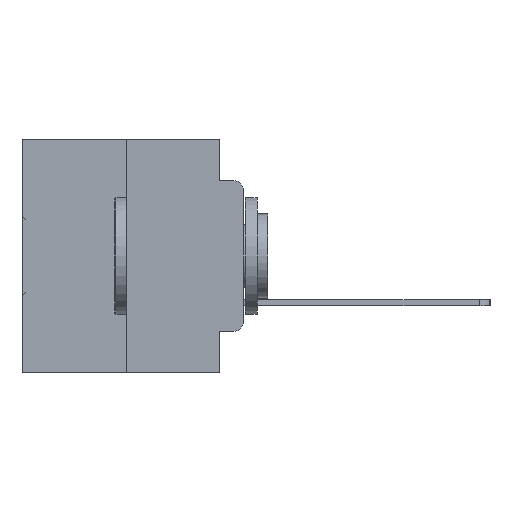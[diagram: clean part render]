
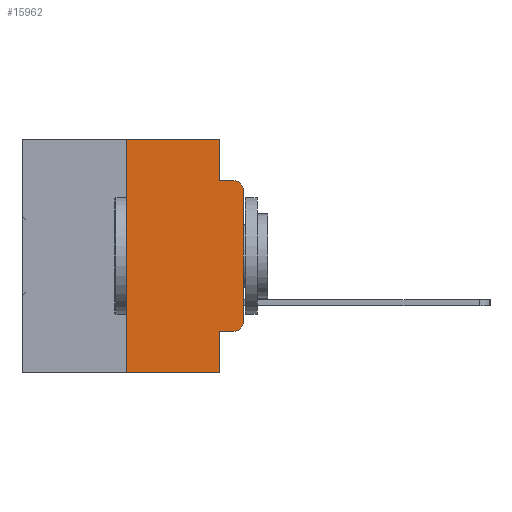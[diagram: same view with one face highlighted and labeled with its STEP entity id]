
A CAD part, left-side view. The second image highlights one B-rep face of the part: STEP entity #15962.
In plain terms, the highlighted planar face has unit normal (-1, 0, 0).
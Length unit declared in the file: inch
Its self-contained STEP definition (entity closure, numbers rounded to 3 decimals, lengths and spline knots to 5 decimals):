
#16 = CARTESIAN_POINT ( 'NONE',  ( 0., 0., 0. ) ) ;
#320 = DIRECTION ( 'NONE',  ( 0., 0., -1. ) ) ;
#1025 = PLANE ( 'NONE',  #18663 ) ;
#1897 = DIRECTION ( 'NONE',  ( 0., -1., 0. ) ) ;
#2776 = AXIS2_PLACEMENT_3D ( 'NONE', #21929, #6407, #24409 ) ;
#3374 = CIRCLE ( 'NONE', #24755, 0.02 ) ;
#3681 = CARTESIAN_POINT ( 'NONE',  ( 0., 0.473, 0. ) ) ;
#3809 = ORIENTED_EDGE ( 'NONE', *, *, #6567, .T. ) ;
#4176 = EDGE_CURVE ( 'NONE', #5156, #12579, #27733, .T. ) ;
#4270 = CARTESIAN_POINT ( 'NONE',  ( 0., 0.02, -0.0885 ) ) ;
#4366 = VECTOR ( 'NONE', #25576, 39.37008 ) ;
#5156 = VERTEX_POINT ( 'NONE', #17436 ) ;
#5177 = LINE ( 'NONE', #10286, #4366 ) ;
#5796 = LINE ( 'NONE', #21014, #32087 ) ;
#5820 = ORIENTED_EDGE ( 'NONE', *, *, #4176, .F. ) ;
#5845 = LINE ( 'NONE', #19561, #12040 ) ;
#6287 = DIRECTION ( 'NONE',  ( 0., 0., -1. ) ) ;
#6336 = CARTESIAN_POINT ( 'NONE',  ( 0., 0.25, -0.5 ) ) ;
#6407 = DIRECTION ( 'NONE',  ( -1., 0., 0. ) ) ;
#6567 = EDGE_CURVE ( 'NONE', #23170, #10672, #9714, .T. ) ;
#6585 = LINE ( 'NONE', #32465, #26214 ) ;
#7095 = CARTESIAN_POINT ( 'NONE',  ( 0., 0.25, 0. ) ) ;
#7705 = EDGE_LOOP ( 'NONE', ( #29774, #10352, #5820, #26272, #15271, #22050, #23598, #30187, #3809, #12429 ) ) ;
#7728 = CARTESIAN_POINT ( 'NONE',  ( 0., 0.051, -0.4115 ) ) ;
#8132 = DIRECTION ( 'NONE',  ( -1., 0., 0. ) ) ;
#9064 = VERTEX_POINT ( 'NONE', #12432 ) ;
#9129 = DIRECTION ( 'NONE',  ( 0., -1., 0. ) ) ;
#9390 = CARTESIAN_POINT ( 'NONE',  ( 0., 0.051, -0.5 ) ) ;
#9714 = LINE ( 'NONE', #30339, #28409 ) ;
#10286 = CARTESIAN_POINT ( 'NONE',  ( 0., 0.25, 0. ) ) ;
#10352 = ORIENTED_EDGE ( 'NONE', *, *, #16430, .T. ) ;
#10590 = DIRECTION ( 'NONE',  ( 0., 0., 1. ) ) ;
#10672 = VERTEX_POINT ( 'NONE', #19319 ) ;
#11258 = VERTEX_POINT ( 'NONE', #9390 ) ;
#11304 = CARTESIAN_POINT ( 'NONE',  ( 0., 0.051, 0. ) ) ;
#12040 = VECTOR ( 'NONE', #9129, 39.37008 ) ;
#12429 = ORIENTED_EDGE ( 'NONE', *, *, #29432, .T. ) ;
#12432 = CARTESIAN_POINT ( 'NONE',  ( 0., 0., -0.1085 ) ) ;
#12579 = VERTEX_POINT ( 'NONE', #4270 ) ;
#13344 = CARTESIAN_POINT ( 'NONE',  ( 0., 0.051, 0. ) ) ;
#14423 = VERTEX_POINT ( 'NONE', #7095 ) ;
#14743 = CARTESIAN_POINT ( 'NONE',  ( 0., 0.051, -0.0885 ) ) ;
#15271 = ORIENTED_EDGE ( 'NONE', *, *, #23002, .F. ) ;
#15962 = ADVANCED_FACE ( 'NONE', ( #23217 ), #1025, .F. ) ;
#16430 = EDGE_CURVE ( 'NONE', #9064, #12579, #3374, .T. ) ;
#16615 = DIRECTION ( 'NONE',  ( 0., 0., -1. ) ) ;
#17080 = EDGE_CURVE ( 'NONE', #23170, #11258, #5796, .T. ) ;
#17436 = CARTESIAN_POINT ( 'NONE',  ( 0., 0.051, -0.0885 ) ) ;
#17939 = VERTEX_POINT ( 'NONE', #6336 ) ;
#18663 = AXIS2_PLACEMENT_3D ( 'NONE', #3681, #21818, #6287 ) ;
#18912 = VECTOR ( 'NONE', #16615, 39.37008 ) ;
#19319 = CARTESIAN_POINT ( 'NONE',  ( 0., 0.02, -0.4115 ) ) ;
#19561 = CARTESIAN_POINT ( 'NONE',  ( 0., 0.473, -0.5 ) ) ;
#19982 = VECTOR ( 'NONE', #10590, 39.37008 ) ;
#21014 = CARTESIAN_POINT ( 'NONE',  ( 0., 0.051, 0. ) ) ;
#21127 = VECTOR ( 'NONE', #32287, 39.37008 ) ;
#21630 = VERTEX_POINT ( 'NONE', #13344 ) ;
#21818 = DIRECTION ( 'NONE',  ( 1., 0., 0. ) ) ;
#21929 = CARTESIAN_POINT ( 'NONE',  ( 0., 0.02, -0.3915 ) ) ;
#22050 = ORIENTED_EDGE ( 'NONE', *, *, #25500, .F. ) ;
#23002 = EDGE_CURVE ( 'NONE', #14423, #21630, #6585, .T. ) ;
#23170 = VERTEX_POINT ( 'NONE', #7728 ) ;
#23217 = FACE_OUTER_BOUND ( 'NONE', #7705, .T. ) ;
#23229 = EDGE_CURVE ( 'NONE', #30530, #9064, #26583, .T. ) ;
#23525 = CARTESIAN_POINT ( 'NONE',  ( 0., 0.02, -0.1085 ) ) ;
#23598 = ORIENTED_EDGE ( 'NONE', *, *, #28506, .T. ) ;
#24409 = DIRECTION ( 'NONE',  ( 0., 0., -1. ) ) ;
#24755 = AXIS2_PLACEMENT_3D ( 'NONE', #23525, #8132, #26004 ) ;
#25500 = EDGE_CURVE ( 'NONE', #17939, #14423, #5177, .T. ) ;
#25576 = DIRECTION ( 'NONE',  ( 0., 0., 1. ) ) ;
#26004 = DIRECTION ( 'NONE',  ( 0., 0., -1. ) ) ;
#26214 = VECTOR ( 'NONE', #1897, 39.37008 ) ;
#26272 = ORIENTED_EDGE ( 'NONE', *, *, #27136, .F. ) ;
#26583 = LINE ( 'NONE', #16, #19982 ) ;
#27136 = EDGE_CURVE ( 'NONE', #21630, #5156, #32940, .T. ) ;
#27733 = LINE ( 'NONE', #14743, #21127 ) ;
#27840 = DIRECTION ( 'NONE',  ( 0., -1., 0. ) ) ;
#28409 = VECTOR ( 'NONE', #27840, 39.37008 ) ;
#28506 = EDGE_CURVE ( 'NONE', #17939, #11258, #5845, .T. ) ;
#29432 = EDGE_CURVE ( 'NONE', #10672, #30530, #32076, .T. ) ;
#29774 = ORIENTED_EDGE ( 'NONE', *, *, #23229, .T. ) ;
#30187 = ORIENTED_EDGE ( 'NONE', *, *, #17080, .F. ) ;
#30339 = CARTESIAN_POINT ( 'NONE',  ( 0., 0.051, -0.4115 ) ) ;
#30530 = VERTEX_POINT ( 'NONE', #31610 ) ;
#31610 = CARTESIAN_POINT ( 'NONE',  ( 0., 0., -0.3915 ) ) ;
#32076 = CIRCLE ( 'NONE', #2776, 0.02 ) ;
#32087 = VECTOR ( 'NONE', #320, 39.37008 ) ;
#32287 = DIRECTION ( 'NONE',  ( 0., -1., 0. ) ) ;
#32465 = CARTESIAN_POINT ( 'NONE',  ( 0., 0.473, 0. ) ) ;
#32940 = LINE ( 'NONE', #11304, #18912 ) ;
